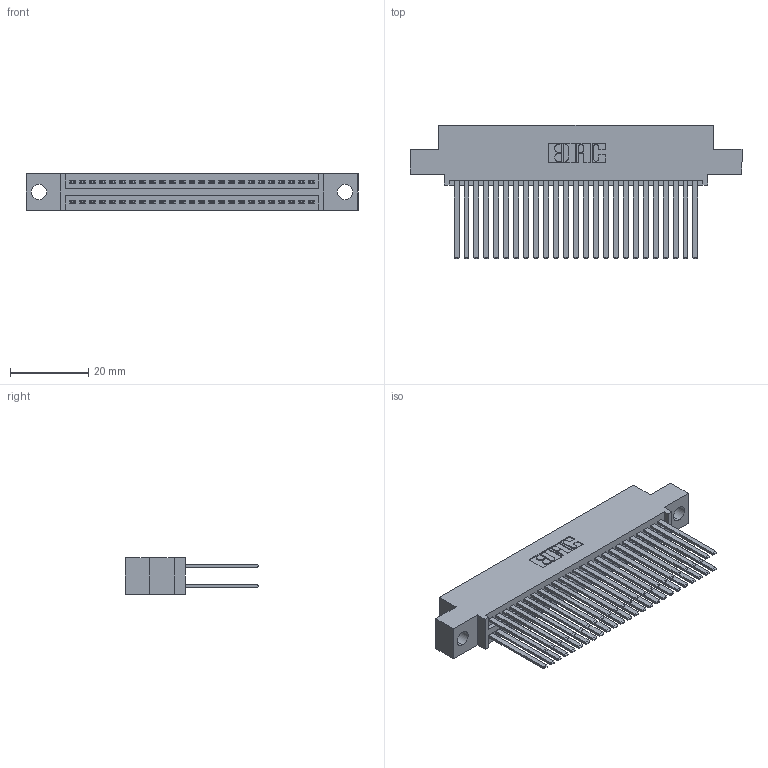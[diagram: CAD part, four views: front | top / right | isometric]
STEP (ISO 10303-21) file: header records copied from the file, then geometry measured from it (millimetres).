
FILE_DESCRIPTION (( 'STEP AP203' ), '1' );
FILE_NAME ('345-050-544-504.STEP', '2021-05-20T03:18:51', ( '' ), ( '' ), 'SwSTEP 2.0', 'SolidWorks 2020', '' );
FILE_SCHEMA (( 'CONFIG_CONTROL_DESIGN' ));
Length unit declared in the file: inch
Products named in the file (3): 345 Part_0.110 Offset - 0.156 Dia-TI; 345-292-001_345-293-144; 345-050-544-504
Assembly tree (51 placements, depth 2):
  345-050-544-504
    345 Part_0.110 Offset - 0.156 Dia-TI
    345-292-001_345-293-144  x50
Bounding box: 84.71 x 33.96 x 9.4 mm (x, y, z)
Volume: 8592.5 mm3; surface area: 14370.6 mm2
Topology: 51 solids, 51 shells, 2344 faces, 6939 edges, 4558 vertices
Faces by surface type: plane 1548, cylinder 796
Entity records: 22271 total; most frequent: CARTESIAN_POINT 3754, ORIENTED_EDGE 3686, DIRECTION 3327, EDGE_CURVE 1843, VECTOR 1615, LINE 1615, VERTEX_POINT 1226, AXIS2_PLACEMENT_3D 856
